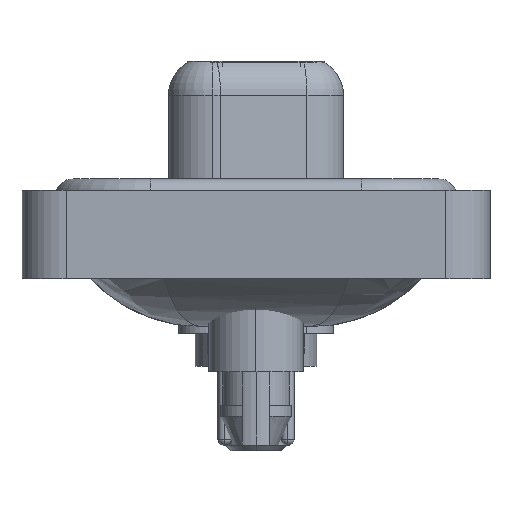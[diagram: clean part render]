
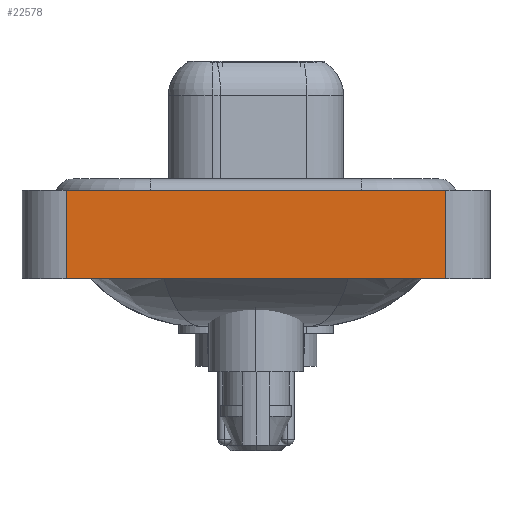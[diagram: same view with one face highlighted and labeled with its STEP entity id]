
A CAD part, left-side view. The second image highlights one B-rep face of the part: STEP entity #22578.
In plain terms, the highlighted planar face has unit normal (-1, 0, 0).
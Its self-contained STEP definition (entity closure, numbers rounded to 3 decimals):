
#45 = LINE ( 'NONE', #10745, #22395 ) ;
#783 = EDGE_LOOP ( 'NONE', ( #925, #23022, #7726, #25137 ) ) ;
#925 = ORIENTED_EDGE ( 'NONE', *, *, #18331, .T. ) ;
#1278 = VECTOR ( 'NONE', #11667, 1000. ) ;
#1726 = CARTESIAN_POINT ( 'NONE',  ( -7.35, 8.55, -3.6 ) ) ;
#2580 = DIRECTION ( 'NONE',  ( 0., -1., 0. ) ) ;
#5548 = VERTEX_POINT ( 'NONE', #22323 ) ;
#7726 = ORIENTED_EDGE ( 'NONE', *, *, #27166, .F. ) ;
#10308 = DIRECTION ( 'NONE',  ( 0., 0., 1. ) ) ;
#10745 = CARTESIAN_POINT ( 'NONE',  ( -7.35, -8.55, -3.6 ) ) ;
#10823 = CARTESIAN_POINT ( 'NONE',  ( -7.35, 8.55, 0.4 ) ) ;
#10977 = FACE_OUTER_BOUND ( 'NONE', #783, .T. ) ;
#11667 = DIRECTION ( 'NONE',  ( 0., -1., 0. ) ) ;
#13906 = LINE ( 'NONE', #22321, #1278 ) ;
#14341 = VECTOR ( 'NONE', #24701, 1000. ) ;
#14518 = LINE ( 'NONE', #1726, #27577 ) ;
#15192 = PLANE ( 'NONE',  #27416 ) ;
#15341 = DIRECTION ( 'NONE',  ( -1., 0., 0. ) ) ;
#16241 = CARTESIAN_POINT ( 'NONE',  ( -7.35, 8.55, -3.6 ) ) ;
#18132 = CARTESIAN_POINT ( 'NONE',  ( -7.35, -8.55, -3.6 ) ) ;
#18331 = EDGE_CURVE ( 'NONE', #5548, #20991, #20498, .T. ) ;
#19408 = DIRECTION ( 'NONE',  ( 0., 0., 1. ) ) ;
#20498 = LINE ( 'NONE', #18132, #14341 ) ;
#20531 = VERTEX_POINT ( 'NONE', #16241 ) ;
#20991 = VERTEX_POINT ( 'NONE', #26989 ) ;
#21367 = EDGE_CURVE ( 'NONE', #26418, #20991, #13906, .T. ) ;
#22321 = CARTESIAN_POINT ( 'NONE',  ( -7.35, -8.55, 0.4 ) ) ;
#22323 = CARTESIAN_POINT ( 'NONE',  ( -7.35, -8.55, -3.6 ) ) ;
#22395 = VECTOR ( 'NONE', #2580, 1000. ) ;
#22578 = ADVANCED_FACE ( 'NONE', ( #10977 ), #15192, .T. ) ;
#23022 = ORIENTED_EDGE ( 'NONE', *, *, #21367, .F. ) ;
#24449 = EDGE_CURVE ( 'NONE', #20531, #5548, #45, .T. ) ;
#24701 = DIRECTION ( 'NONE',  ( 0., 0., 1. ) ) ;
#25137 = ORIENTED_EDGE ( 'NONE', *, *, #24449, .T. ) ;
#26274 = CARTESIAN_POINT ( 'NONE',  ( -7.35, -8.55, -3.6 ) ) ;
#26418 = VERTEX_POINT ( 'NONE', #10823 ) ;
#26989 = CARTESIAN_POINT ( 'NONE',  ( -7.35, -8.55, 0.4 ) ) ;
#27166 = EDGE_CURVE ( 'NONE', #20531, #26418, #14518, .T. ) ;
#27416 = AXIS2_PLACEMENT_3D ( 'NONE', #26274, #15341, #19408 ) ;
#27577 = VECTOR ( 'NONE', #10308, 1000. ) ;
